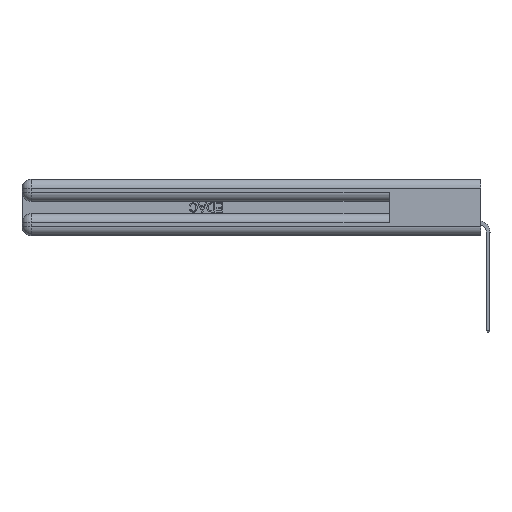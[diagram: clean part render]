
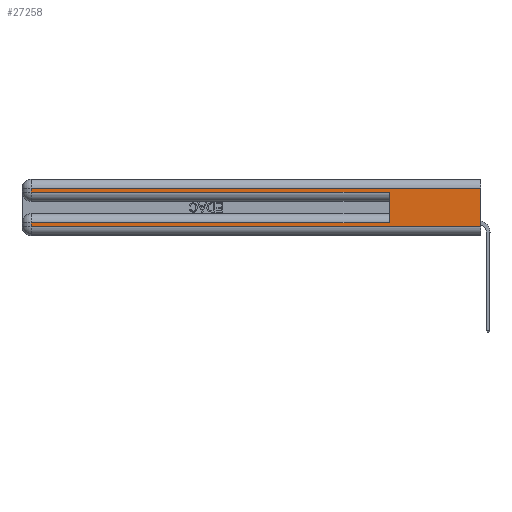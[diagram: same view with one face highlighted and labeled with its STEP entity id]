
A CAD part, left-side view. The second image highlights one B-rep face of the part: STEP entity #27258.
In plain terms, the highlighted planar face has unit normal (-1, 0, 0).
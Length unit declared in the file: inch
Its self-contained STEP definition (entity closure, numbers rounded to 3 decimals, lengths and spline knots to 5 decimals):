
#1 = ORIENTED_EDGE ( 'NONE', *, *, #32094, .T. ) ;
#443 = VERTEX_POINT ( 'NONE', #17127 ) ;
#450 = DIRECTION ( 'NONE',  ( 0., 0., -1. ) ) ;
#1558 = VERTEX_POINT ( 'NONE', #30597 ) ;
#2176 = CARTESIAN_POINT ( 'NONE',  ( 0., 0., 0.085 ) ) ;
#5255 = LINE ( 'NONE', #32158, #31822 ) ;
#7545 = EDGE_CURVE ( 'NONE', #443, #37277, #37673, .T. ) ;
#9214 = EDGE_CURVE ( 'NONE', #33924, #1558, #42823, .T. ) ;
#10336 = ORIENTED_EDGE ( 'NONE', *, *, #35789, .T. ) ;
#11099 = EDGE_LOOP ( 'NONE', ( #18095, #10336, #1, #43267, #11551, #17459, #20034, #41509 ) ) ;
#11551 = ORIENTED_EDGE ( 'NONE', *, *, #38543, .F. ) ;
#11853 = CARTESIAN_POINT ( 'NONE',  ( 0., 0., 0.285 ) ) ;
#12229 = CARTESIAN_POINT ( 'NONE',  ( 0., 0.6, 0.285 ) ) ;
#13041 = VERTEX_POINT ( 'NONE', #12229 ) ;
#13085 = LINE ( 'NONE', #2176, #27771 ) ;
#15348 = CARTESIAN_POINT ( 'NONE',  ( 0., 0., 0.37 ) ) ;
#15390 = VECTOR ( 'NONE', #32456, 39.37008 ) ;
#16021 = VERTEX_POINT ( 'NONE', #25524 ) ;
#16259 = CARTESIAN_POINT ( 'NONE',  ( 0., 2.94, 0.37 ) ) ;
#16530 = LINE ( 'NONE', #36078, #15390 ) ;
#16582 = EDGE_CURVE ( 'NONE', #1558, #37277, #16530, .T. ) ;
#17127 = CARTESIAN_POINT ( 'NONE',  ( 0., 0., 0.31 ) ) ;
#17459 = ORIENTED_EDGE ( 'NONE', *, *, #33372, .T. ) ;
#17502 = VECTOR ( 'NONE', #23409, 39.37008 ) ;
#18095 = ORIENTED_EDGE ( 'NONE', *, *, #7545, .F. ) ;
#18465 = LINE ( 'NONE', #30513, #27271 ) ;
#18846 = DIRECTION ( 'NONE',  ( 0., 0., -1. ) ) ;
#20034 = ORIENTED_EDGE ( 'NONE', *, *, #9214, .T. ) ;
#20985 = AXIS2_PLACEMENT_3D ( 'NONE', #15348, #39670, #18846 ) ;
#22887 = CARTESIAN_POINT ( 'NONE',  ( 0., 2.94, 0.37 ) ) ;
#23397 = CARTESIAN_POINT ( 'NONE',  ( 0., 2.94, 0.285 ) ) ;
#23409 = DIRECTION ( 'NONE',  ( 0., 0., -1. ) ) ;
#25524 = CARTESIAN_POINT ( 'NONE',  ( 0., 0.6, 0.085 ) ) ;
#27258 = ADVANCED_FACE ( 'NONE', ( #41366 ), #36166, .F. ) ;
#27271 = VECTOR ( 'NONE', #33847, 39.37008 ) ;
#27771 = VECTOR ( 'NONE', #34282, 39.37008 ) ;
#27970 = VECTOR ( 'NONE', #42744, 39.37008 ) ;
#30513 = CARTESIAN_POINT ( 'NONE',  ( 0., 0.6, 0.145 ) ) ;
#30597 = CARTESIAN_POINT ( 'NONE',  ( 0., 2.94, 0.06 ) ) ;
#31094 = EDGE_CURVE ( 'NONE', #43297, #13041, #36648, .T. ) ;
#31151 = LINE ( 'NONE', #16259, #17502 ) ;
#31647 = CARTESIAN_POINT ( 'NONE',  ( 0., 0., 0.37 ) ) ;
#31791 = CARTESIAN_POINT ( 'NONE',  ( 0., 2.94, 0.085 ) ) ;
#31822 = VECTOR ( 'NONE', #35195, 39.37008 ) ;
#32094 = EDGE_CURVE ( 'NONE', #37134, #43297, #31151, .T. ) ;
#32158 = CARTESIAN_POINT ( 'NONE',  ( 0., 0., 0.31 ) ) ;
#32456 = DIRECTION ( 'NONE',  ( 0., -1., 0. ) ) ;
#33372 = EDGE_CURVE ( 'NONE', #16021, #33924, #13085, .T. ) ;
#33847 = DIRECTION ( 'NONE',  ( 0., 0., 1. ) ) ;
#33924 = VERTEX_POINT ( 'NONE', #31791 ) ;
#34282 = DIRECTION ( 'NONE',  ( 0., 1., 0. ) ) ;
#34403 = VECTOR ( 'NONE', #450, 39.37008 ) ;
#34811 = DIRECTION ( 'NONE',  ( 0., 0., -1. ) ) ;
#35195 = DIRECTION ( 'NONE',  ( 0., 1., 0. ) ) ;
#35789 = EDGE_CURVE ( 'NONE', #443, #37134, #5255, .T. ) ;
#35791 = VECTOR ( 'NONE', #34811, 39.37008 ) ;
#35889 = CARTESIAN_POINT ( 'NONE',  ( 0., 0., 0.06 ) ) ;
#36078 = CARTESIAN_POINT ( 'NONE',  ( 0., 0., 0.06 ) ) ;
#36166 = PLANE ( 'NONE',  #20985 ) ;
#36648 = LINE ( 'NONE', #11853, #27970 ) ;
#37134 = VERTEX_POINT ( 'NONE', #38808 ) ;
#37277 = VERTEX_POINT ( 'NONE', #35889 ) ;
#37673 = LINE ( 'NONE', #31647, #34403 ) ;
#38543 = EDGE_CURVE ( 'NONE', #16021, #13041, #18465, .T. ) ;
#38808 = CARTESIAN_POINT ( 'NONE',  ( 0., 2.94, 0.31 ) ) ;
#39670 = DIRECTION ( 'NONE',  ( 1., 0., 0. ) ) ;
#41366 = FACE_OUTER_BOUND ( 'NONE', #11099, .T. ) ;
#41509 = ORIENTED_EDGE ( 'NONE', *, *, #16582, .T. ) ;
#42744 = DIRECTION ( 'NONE',  ( 0., -1., 0. ) ) ;
#42823 = LINE ( 'NONE', #22887, #35791 ) ;
#43267 = ORIENTED_EDGE ( 'NONE', *, *, #31094, .T. ) ;
#43297 = VERTEX_POINT ( 'NONE', #23397 ) ;
